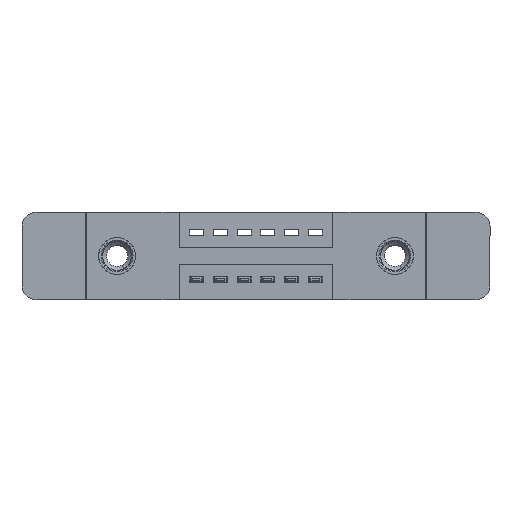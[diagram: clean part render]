
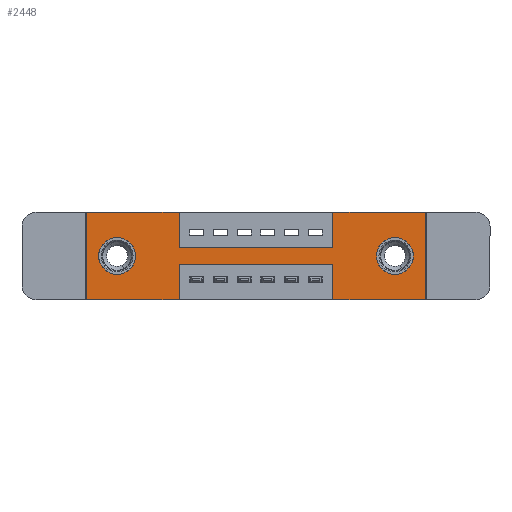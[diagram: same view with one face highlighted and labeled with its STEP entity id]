
A CAD part, front view. The second image highlights one B-rep face of the part: STEP entity #2448.
In plain terms, the highlighted planar face has unit normal (0, -1, 0).
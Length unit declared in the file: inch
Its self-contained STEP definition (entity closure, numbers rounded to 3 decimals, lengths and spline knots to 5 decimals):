
#167 = CARTESIAN_POINT ( 'NONE',  ( 0.13, 0., -0.107 ) ) ;
#184 = CARTESIAN_POINT ( 'NONE',  ( 0., 0., 0. ) ) ;
#206 = VERTEX_POINT ( 'NONE', #9127 ) ;
#211 = CARTESIAN_POINT ( 'NONE',  ( 1.0425, 0., -0.37 ) ) ;
#312 = VECTOR ( 'NONE', #10054, 39.37008 ) ;
#345 = DIRECTION ( 'NONE',  ( 0., 0., 1. ) ) ;
#444 = EDGE_CURVE ( 'NONE', #8771, #206, #10403, .T. ) ;
#495 = DIRECTION ( 'NONE',  ( -1., 0., 0. ) ) ;
#701 = ORIENTED_EDGE ( 'NONE', *, *, #7223, .T. ) ;
#1021 = VECTOR ( 'NONE', #10344, 39.37008 ) ;
#1067 = ORIENTED_EDGE ( 'NONE', *, *, #13497, .F. ) ;
#1274 = DIRECTION ( 'NONE',  ( 0., 0., -1. ) ) ;
#1312 = VECTOR ( 'NONE', #7926, 39.37008 ) ;
#1568 = LINE ( 'NONE', #7411, #1919 ) ;
#1589 = EDGE_LOOP ( 'NONE', ( #701, #6229 ) ) ;
#1605 = DIRECTION ( 'NONE',  ( 0., 0., -1. ) ) ;
#1658 = EDGE_CURVE ( 'NONE', #2387, #8077, #4462, .T. ) ;
#1687 = CARTESIAN_POINT ( 'NONE',  ( 0., 0., -0.37 ) ) ;
#1755 = CARTESIAN_POINT ( 'NONE',  ( 1.305, 0., -0.185 ) ) ;
#1919 = VECTOR ( 'NONE', #8562, 39.37008 ) ;
#1991 = DIRECTION ( 'NONE',  ( 0., 0., -1. ) ) ;
#2036 = DIRECTION ( 'NONE',  ( 0., 1., 0. ) ) ;
#2100 = EDGE_CURVE ( 'NONE', #4025, #3869, #2759, .T. ) ;
#2387 = VERTEX_POINT ( 'NONE', #9455 ) ;
#2436 = CARTESIAN_POINT ( 'NONE',  ( 1.435, 0., 0. ) ) ;
#2448 = ADVANCED_FACE ( 'NONE', ( #4465, #10541, #7058 ), #8500, .T. ) ;
#2511 = ORIENTED_EDGE ( 'NONE', *, *, #3647, .T. ) ;
#2609 = CARTESIAN_POINT ( 'NONE',  ( 1.0425, 0., -0.37 ) ) ;
#2614 = DIRECTION ( 'NONE',  ( -1., 0., 0. ) ) ;
#2669 = EDGE_LOOP ( 'NONE', ( #14332, #2511 ) ) ;
#2684 = ORIENTED_EDGE ( 'NONE', *, *, #1658, .F. ) ;
#2727 = LINE ( 'NONE', #2609, #8244 ) ;
#2759 = LINE ( 'NONE', #11969, #11233 ) ;
#2793 = EDGE_CURVE ( 'NONE', #4267, #12525, #7045, .T. ) ;
#2797 = CIRCLE ( 'NONE', #4566, 0.078 ) ;
#2858 = EDGE_LOOP ( 'NONE', ( #6047, #13723, #11913, #3006, #6748, #5586, #2684, #9607, #1067, #9241, #10807, #6376 ) ) ;
#2925 = CIRCLE ( 'NONE', #9716, 0.078 ) ;
#3006 = ORIENTED_EDGE ( 'NONE', *, *, #4824, .F. ) ;
#3347 = EDGE_CURVE ( 'NONE', #8855, #2387, #4087, .T. ) ;
#3380 = DIRECTION ( 'NONE',  ( 0., 0., 1. ) ) ;
#3647 = EDGE_CURVE ( 'NONE', #4406, #14290, #6226, .T. ) ;
#3695 = CARTESIAN_POINT ( 'NONE',  ( 0., 0., -0.37 ) ) ;
#3699 = CARTESIAN_POINT ( 'NONE',  ( 0., 0., -0.37 ) ) ;
#3869 = VERTEX_POINT ( 'NONE', #4296 ) ;
#4025 = VERTEX_POINT ( 'NONE', #4595 ) ;
#4087 = LINE ( 'NONE', #9042, #1312 ) ;
#4109 = LINE ( 'NONE', #11212, #312 ) ;
#4112 = DIRECTION ( 'NONE',  ( 0., -1., 0. ) ) ;
#4267 = VERTEX_POINT ( 'NONE', #7203 ) ;
#4296 = CARTESIAN_POINT ( 'NONE',  ( 0.3925, 0., 0. ) ) ;
#4406 = VERTEX_POINT ( 'NONE', #5856 ) ;
#4462 = LINE ( 'NONE', #13403, #5165 ) ;
#4465 = FACE_BOUND ( 'NONE', #2669, .T. ) ;
#4566 = AXIS2_PLACEMENT_3D ( 'NONE', #1755, #7268, #1605 ) ;
#4595 = CARTESIAN_POINT ( 'NONE',  ( 0., 0., 0. ) ) ;
#4689 = LINE ( 'NONE', #3695, #9691 ) ;
#4741 = LINE ( 'NONE', #6991, #7324 ) ;
#4815 = VECTOR ( 'NONE', #2614, 39.37008 ) ;
#4824 = EDGE_CURVE ( 'NONE', #206, #12634, #4689, .T. ) ;
#5165 = VECTOR ( 'NONE', #7823, 39.37008 ) ;
#5320 = VERTEX_POINT ( 'NONE', #6655 ) ;
#5352 = EDGE_CURVE ( 'NONE', #12525, #4025, #11447, .T. ) ;
#5586 = ORIENTED_EDGE ( 'NONE', *, *, #11709, .F. ) ;
#5652 = VECTOR ( 'NONE', #8399, 39.37008 ) ;
#5856 = CARTESIAN_POINT ( 'NONE',  ( 1.305, 0., -0.263 ) ) ;
#5867 = VECTOR ( 'NONE', #3380, 39.37008 ) ;
#6047 = ORIENTED_EDGE ( 'NONE', *, *, #10179, .F. ) ;
#6113 = AXIS2_PLACEMENT_3D ( 'NONE', #13208, #2036, #7668 ) ;
#6226 = CIRCLE ( 'NONE', #14099, 0.078 ) ;
#6229 = ORIENTED_EDGE ( 'NONE', *, *, #6638, .T. ) ;
#6376 = ORIENTED_EDGE ( 'NONE', *, *, #2793, .F. ) ;
#6638 = EDGE_CURVE ( 'NONE', #7649, #14276, #2925, .T. ) ;
#6655 = CARTESIAN_POINT ( 'NONE',  ( 0.3925, 0., -0.22 ) ) ;
#6748 = ORIENTED_EDGE ( 'NONE', *, *, #444, .F. ) ;
#6919 = DIRECTION ( 'NONE',  ( 0., 1., 0. ) ) ;
#6991 = CARTESIAN_POINT ( 'NONE',  ( 0.3925, 0., -0.37 ) ) ;
#7045 = LINE ( 'NONE', #1687, #4815 ) ;
#7058 = FACE_OUTER_BOUND ( 'NONE', #2858, .T. ) ;
#7203 = CARTESIAN_POINT ( 'NONE',  ( 0.3925, 0., -0.37 ) ) ;
#7223 = EDGE_CURVE ( 'NONE', #14276, #7649, #12775, .T. ) ;
#7268 = DIRECTION ( 'NONE',  ( 0., 1., 0. ) ) ;
#7324 = VECTOR ( 'NONE', #8096, 39.37008 ) ;
#7386 = CARTESIAN_POINT ( 'NONE',  ( 0.3925, 0., -0.15 ) ) ;
#7411 = CARTESIAN_POINT ( 'NONE',  ( 0., 0., 0. ) ) ;
#7418 = EDGE_CURVE ( 'NONE', #12634, #11809, #2727, .T. ) ;
#7649 = VERTEX_POINT ( 'NONE', #13152 ) ;
#7668 = DIRECTION ( 'NONE',  ( 0., 0., 1. ) ) ;
#7747 = LINE ( 'NONE', #13865, #5652 ) ;
#7823 = DIRECTION ( 'NONE',  ( 0., 0., 1. ) ) ;
#7926 = DIRECTION ( 'NONE',  ( 1., 0., 0. ) ) ;
#8077 = VERTEX_POINT ( 'NONE', #13920 ) ;
#8085 = CARTESIAN_POINT ( 'NONE',  ( 1.0425, 0., -0.22 ) ) ;
#8096 = DIRECTION ( 'NONE',  ( 0., 0., -1. ) ) ;
#8244 = VECTOR ( 'NONE', #11260, 39.37008 ) ;
#8399 = DIRECTION ( 'NONE',  ( 0., 0., -1. ) ) ;
#8500 = PLANE ( 'NONE',  #14081 ) ;
#8562 = DIRECTION ( 'NONE',  ( 1., 0., 0. ) ) ;
#8771 = VERTEX_POINT ( 'NONE', #13524 ) ;
#8855 = VERTEX_POINT ( 'NONE', #7386 ) ;
#9042 = CARTESIAN_POINT ( 'NONE',  ( 0.3925, 0., -0.15 ) ) ;
#9075 = DIRECTION ( 'NONE',  ( 0., 1., 0. ) ) ;
#9127 = CARTESIAN_POINT ( 'NONE',  ( 1.435, 0., -0.37 ) ) ;
#9241 = ORIENTED_EDGE ( 'NONE', *, *, #2100, .F. ) ;
#9455 = CARTESIAN_POINT ( 'NONE',  ( 1.0425, 0., -0.15 ) ) ;
#9607 = ORIENTED_EDGE ( 'NONE', *, *, #3347, .F. ) ;
#9691 = VECTOR ( 'NONE', #495, 39.37008 ) ;
#9716 = AXIS2_PLACEMENT_3D ( 'NONE', #12455, #6919, #345 ) ;
#10054 = DIRECTION ( 'NONE',  ( -1., 0., 0. ) ) ;
#10179 = EDGE_CURVE ( 'NONE', #5320, #4267, #4741, .T. ) ;
#10344 = DIRECTION ( 'NONE',  ( 0., 0., -1. ) ) ;
#10403 = LINE ( 'NONE', #2436, #1021 ) ;
#10541 = FACE_BOUND ( 'NONE', #1589, .T. ) ;
#10807 = ORIENTED_EDGE ( 'NONE', *, *, #5352, .F. ) ;
#10935 = CARTESIAN_POINT ( 'NONE',  ( 0., 0., -0.37 ) ) ;
#11212 = CARTESIAN_POINT ( 'NONE',  ( 0.3925, 0., -0.22 ) ) ;
#11233 = VECTOR ( 'NONE', #12984, 39.37008 ) ;
#11260 = DIRECTION ( 'NONE',  ( 0., 0., 1. ) ) ;
#11423 = CARTESIAN_POINT ( 'NONE',  ( 1.305, 0., -0.185 ) ) ;
#11447 = LINE ( 'NONE', #184, #5867 ) ;
#11709 = EDGE_CURVE ( 'NONE', #8077, #8771, #1568, .T. ) ;
#11809 = VERTEX_POINT ( 'NONE', #8085 ) ;
#11861 = EDGE_CURVE ( 'NONE', #14290, #4406, #2797, .T. ) ;
#11913 = ORIENTED_EDGE ( 'NONE', *, *, #7418, .F. ) ;
#11969 = CARTESIAN_POINT ( 'NONE',  ( 0., 0., 0. ) ) ;
#12363 = CARTESIAN_POINT ( 'NONE',  ( 1.305, 0., -0.107 ) ) ;
#12455 = CARTESIAN_POINT ( 'NONE',  ( 0.13, 0., -0.185 ) ) ;
#12525 = VERTEX_POINT ( 'NONE', #3699 ) ;
#12634 = VERTEX_POINT ( 'NONE', #211 ) ;
#12775 = CIRCLE ( 'NONE', #6113, 0.078 ) ;
#12984 = DIRECTION ( 'NONE',  ( 1., 0., 0. ) ) ;
#13152 = CARTESIAN_POINT ( 'NONE',  ( 0.13, 0., -0.263 ) ) ;
#13208 = CARTESIAN_POINT ( 'NONE',  ( 0.13, 0., -0.185 ) ) ;
#13403 = CARTESIAN_POINT ( 'NONE',  ( 1.0425, 0., 0. ) ) ;
#13497 = EDGE_CURVE ( 'NONE', #3869, #8855, #7747, .T. ) ;
#13524 = CARTESIAN_POINT ( 'NONE',  ( 1.435, 0., 0. ) ) ;
#13723 = ORIENTED_EDGE ( 'NONE', *, *, #13748, .F. ) ;
#13748 = EDGE_CURVE ( 'NONE', #11809, #5320, #4109, .T. ) ;
#13865 = CARTESIAN_POINT ( 'NONE',  ( 0.3925, 0., 0. ) ) ;
#13920 = CARTESIAN_POINT ( 'NONE',  ( 1.0425, 0., 0. ) ) ;
#14081 = AXIS2_PLACEMENT_3D ( 'NONE', #10935, #4112, #1991 ) ;
#14099 = AXIS2_PLACEMENT_3D ( 'NONE', #11423, #9075, #1274 ) ;
#14276 = VERTEX_POINT ( 'NONE', #167 ) ;
#14290 = VERTEX_POINT ( 'NONE', #12363 ) ;
#14332 = ORIENTED_EDGE ( 'NONE', *, *, #11861, .T. ) ;
